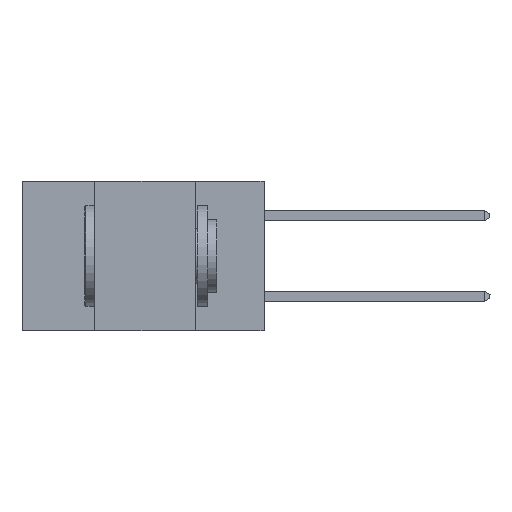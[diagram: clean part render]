
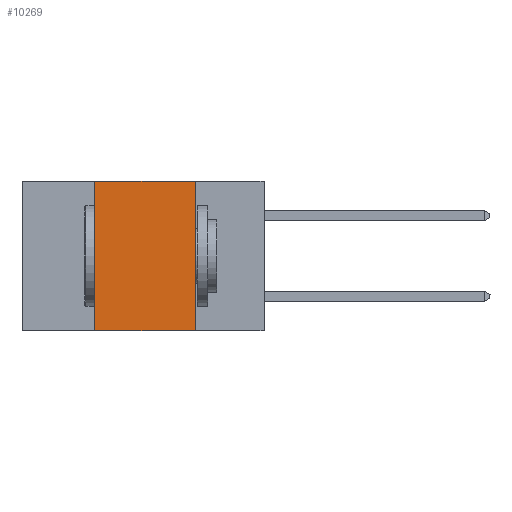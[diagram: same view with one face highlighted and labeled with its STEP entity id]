
A CAD part, left-side view. The second image highlights one B-rep face of the part: STEP entity #10269.
In plain terms, the highlighted planar face has unit normal (-1, 0, 0).
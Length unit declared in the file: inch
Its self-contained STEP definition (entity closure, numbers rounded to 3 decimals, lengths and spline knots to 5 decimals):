
#111 = PLANE ( 'NONE',  #16430 ) ;
#123 = VERTEX_POINT ( 'NONE', #14743 ) ;
#1991 = DIRECTION ( 'NONE',  ( 1., 0., 0. ) ) ;
#2601 = LINE ( 'NONE', #12654, #21952 ) ;
#3748 = CARTESIAN_POINT ( 'NONE',  ( 0., 0.6, 0. ) ) ;
#5425 = CARTESIAN_POINT ( 'NONE',  ( 0., 0.42, -0.37 ) ) ;
#5889 = LINE ( 'NONE', #3748, #15948 ) ;
#6225 = CARTESIAN_POINT ( 'NONE',  ( 0., 0.42, -0.37 ) ) ;
#6423 = VERTEX_POINT ( 'NONE', #6225 ) ;
#8821 = DIRECTION ( 'NONE',  ( 0., -1., 0. ) ) ;
#8880 = EDGE_CURVE ( 'NONE', #6423, #123, #14707, .T. ) ;
#8939 = EDGE_LOOP ( 'NONE', ( #22490, #9013, #17525, #10845 ) ) ;
#9013 = ORIENTED_EDGE ( 'NONE', *, *, #14761, .F. ) ;
#10269 = ADVANCED_FACE ( 'NONE', ( #13470 ), #111, .F. ) ;
#10845 = ORIENTED_EDGE ( 'NONE', *, *, #17655, .T. ) ;
#10980 = DIRECTION ( 'NONE',  ( 0., 0., -1. ) ) ;
#11335 = CARTESIAN_POINT ( 'NONE',  ( 0., 0.6, 0. ) ) ;
#12654 = CARTESIAN_POINT ( 'NONE',  ( 0., 0.6, -0.37 ) ) ;
#12824 = VERTEX_POINT ( 'NONE', #16760 ) ;
#13470 = FACE_OUTER_BOUND ( 'NONE', #8939, .T. ) ;
#14288 = VECTOR ( 'NONE', #10980, 39.37008 ) ;
#14707 = LINE ( 'NONE', #5425, #18496 ) ;
#14743 = CARTESIAN_POINT ( 'NONE',  ( 0., 0.42, 0. ) ) ;
#14761 = EDGE_CURVE ( 'NONE', #123, #12824, #5889, .T. ) ;
#15039 = DIRECTION ( 'NONE',  ( 0., -1., 0. ) ) ;
#15138 = DIRECTION ( 'NONE',  ( 0., 0., -1. ) ) ;
#15948 = VECTOR ( 'NONE', #15039, 39.37008 ) ;
#16430 = AXIS2_PLACEMENT_3D ( 'NONE', #11335, #1991, #15138 ) ;
#16760 = CARTESIAN_POINT ( 'NONE',  ( 0., 0.17, 0. ) ) ;
#17525 = ORIENTED_EDGE ( 'NONE', *, *, #8880, .F. ) ;
#17655 = EDGE_CURVE ( 'NONE', #6423, #20753, #2601, .T. ) ;
#18496 = VECTOR ( 'NONE', #18611, 39.37008 ) ;
#18611 = DIRECTION ( 'NONE',  ( 0., 0., 1. ) ) ;
#18682 = CARTESIAN_POINT ( 'NONE',  ( 0., 0.17, -0.37 ) ) ;
#19235 = LINE ( 'NONE', #20319, #14288 ) ;
#19802 = EDGE_CURVE ( 'NONE', #12824, #20753, #19235, .T. ) ;
#20319 = CARTESIAN_POINT ( 'NONE',  ( 0., 0.17, -0.37 ) ) ;
#20753 = VERTEX_POINT ( 'NONE', #18682 ) ;
#21952 = VECTOR ( 'NONE', #8821, 39.37008 ) ;
#22490 = ORIENTED_EDGE ( 'NONE', *, *, #19802, .F. ) ;
